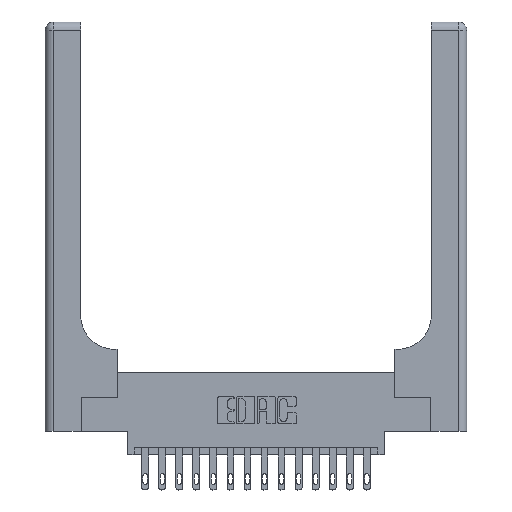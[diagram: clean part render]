
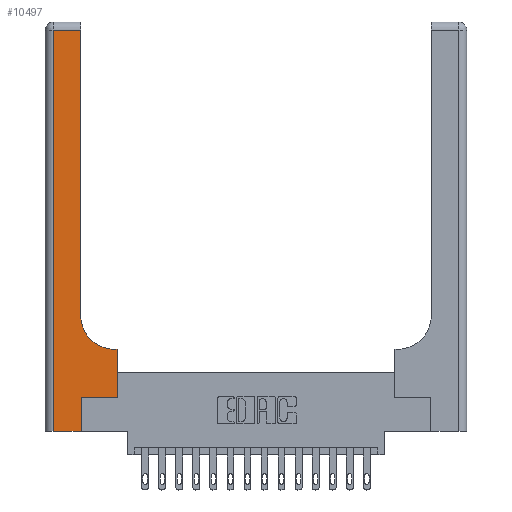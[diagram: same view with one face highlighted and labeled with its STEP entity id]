
A CAD part, top view. The second image highlights one B-rep face of the part: STEP entity #10497.
In plain terms, the highlighted planar face has unit normal (0, 0, 1).
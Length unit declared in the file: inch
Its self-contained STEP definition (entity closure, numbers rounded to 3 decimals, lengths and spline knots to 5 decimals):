
#294 = DIRECTION ( 'NONE',  ( -1., 0., 0. ) ) ;
#626 = LINE ( 'NONE', #2145, #14261 ) ;
#1012 = EDGE_CURVE ( 'NONE', #3552, #9337, #626, .T. ) ;
#1110 = VERTEX_POINT ( 'NONE', #9765 ) ;
#1452 = EDGE_CURVE ( 'NONE', #13508, #1110, #2634, .T. ) ;
#1680 = VECTOR ( 'NONE', #11181, 39.37008 ) ;
#2010 = EDGE_CURVE ( 'NONE', #9337, #5900, #4850, .T. ) ;
#2100 = VECTOR ( 'NONE', #17660, 39.37008 ) ;
#2145 = CARTESIAN_POINT ( 'NONE',  ( 0.06, 3., 0.37 ) ) ;
#2224 = AXIS2_PLACEMENT_3D ( 'NONE', #9870, #9687, #8454 ) ;
#2429 = CARTESIAN_POINT ( 'NONE',  ( 0., 3., 0.37 ) ) ;
#2634 = LINE ( 'NONE', #2726, #1680 ) ;
#2726 = CARTESIAN_POINT ( 'NONE',  ( 0.528, 0.25, 0.37 ) ) ;
#2947 = CARTESIAN_POINT ( 'NONE',  ( 0., 2.94, 0.37 ) ) ;
#3294 = VECTOR ( 'NONE', #8867, 39.37008 ) ;
#3315 = DIRECTION ( 'NONE',  ( -1., 0., 0. ) ) ;
#3552 = VERTEX_POINT ( 'NONE', #4098 ) ;
#3601 = CARTESIAN_POINT ( 'NONE',  ( 0.51, 0.6, 0.37 ) ) ;
#3669 = EDGE_CURVE ( 'NONE', #10164, #10861, #8691, .T. ) ;
#3693 = CARTESIAN_POINT ( 'NONE',  ( 0.26, 0.6, 0.37 ) ) ;
#4098 = CARTESIAN_POINT ( 'NONE',  ( 0.06, 2.94, 0.37 ) ) ;
#4128 = PLANE ( 'NONE',  #4860 ) ;
#4425 = CARTESIAN_POINT ( 'NONE',  ( 0.265, 0., 0.37 ) ) ;
#4574 = CARTESIAN_POINT ( 'NONE',  ( 0.265, 0.25, 0.37 ) ) ;
#4850 = LINE ( 'NONE', #15861, #9559 ) ;
#4860 = AXIS2_PLACEMENT_3D ( 'NONE', #2429, #15585, #13957 ) ;
#5301 = EDGE_CURVE ( 'NONE', #1110, #5337, #7560, .T. ) ;
#5337 = VERTEX_POINT ( 'NONE', #3601 ) ;
#5899 = EDGE_CURVE ( 'NONE', #11360, #13508, #14433, .T. ) ;
#5900 = VERTEX_POINT ( 'NONE', #10310 ) ;
#6257 = ORIENTED_EDGE ( 'NONE', *, *, #1012, .T. ) ;
#6306 = VECTOR ( 'NONE', #294, 39.37008 ) ;
#6399 = ORIENTED_EDGE ( 'NONE', *, *, #1452, .T. ) ;
#6915 = EDGE_LOOP ( 'NONE', ( #8743, #10645, #6257, #13335, #11617, #18460, #6399, #18344, #11744 ) ) ;
#7560 = LINE ( 'NONE', #3693, #11425 ) ;
#7671 = DIRECTION ( 'NONE',  ( 1., 0., 0. ) ) ;
#8454 = DIRECTION ( 'NONE',  ( 1., 0., 0. ) ) ;
#8691 = LINE ( 'NONE', #14410, #3294 ) ;
#8743 = ORIENTED_EDGE ( 'NONE', *, *, #3669, .T. ) ;
#8867 = DIRECTION ( 'NONE',  ( 0., 1., 0. ) ) ;
#9084 = CARTESIAN_POINT ( 'NONE',  ( 0.528, 0.25, 0.37 ) ) ;
#9337 = VERTEX_POINT ( 'NONE', #11596 ) ;
#9559 = VECTOR ( 'NONE', #10400, 39.37008 ) ;
#9687 = DIRECTION ( 'NONE',  ( 0., 0., -1. ) ) ;
#9765 = CARTESIAN_POINT ( 'NONE',  ( 0.528, 0.6, 0.37 ) ) ;
#9870 = CARTESIAN_POINT ( 'NONE',  ( 0.51, 0.85, 0.37 ) ) ;
#10066 = CARTESIAN_POINT ( 'NONE',  ( 0.265, 0.25, 0.37 ) ) ;
#10164 = VERTEX_POINT ( 'NONE', #10249 ) ;
#10249 = CARTESIAN_POINT ( 'NONE',  ( 0.26, 0.85, 0.37 ) ) ;
#10310 = CARTESIAN_POINT ( 'NONE',  ( 0.265, 0., 0.37 ) ) ;
#10342 = CIRCLE ( 'NONE', #2224, 0.25 ) ;
#10400 = DIRECTION ( 'NONE',  ( 1., 0., 0. ) ) ;
#10497 = ADVANCED_FACE ( 'NONE', ( #12645 ), #4128, .F. ) ;
#10645 = ORIENTED_EDGE ( 'NONE', *, *, #12958, .T. ) ;
#10861 = VERTEX_POINT ( 'NONE', #13758 ) ;
#11181 = DIRECTION ( 'NONE',  ( 0., 1., 0. ) ) ;
#11360 = VERTEX_POINT ( 'NONE', #10066 ) ;
#11425 = VECTOR ( 'NONE', #3315, 39.37008 ) ;
#11560 = EDGE_CURVE ( 'NONE', #5900, #11360, #13310, .T. ) ;
#11596 = CARTESIAN_POINT ( 'NONE',  ( 0.06, 0., 0.37 ) ) ;
#11617 = ORIENTED_EDGE ( 'NONE', *, *, #11560, .T. ) ;
#11744 = ORIENTED_EDGE ( 'NONE', *, *, #16178, .T. ) ;
#12645 = FACE_OUTER_BOUND ( 'NONE', #6915, .T. ) ;
#12958 = EDGE_CURVE ( 'NONE', #10861, #3552, #17139, .T. ) ;
#13310 = LINE ( 'NONE', #4425, #2100 ) ;
#13335 = ORIENTED_EDGE ( 'NONE', *, *, #2010, .T. ) ;
#13508 = VERTEX_POINT ( 'NONE', #9084 ) ;
#13679 = DIRECTION ( 'NONE',  ( 0., -1., 0. ) ) ;
#13758 = CARTESIAN_POINT ( 'NONE',  ( 0.26, 2.94, 0.37 ) ) ;
#13957 = DIRECTION ( 'NONE',  ( -1., 0., 0. ) ) ;
#14261 = VECTOR ( 'NONE', #13679, 39.37008 ) ;
#14410 = CARTESIAN_POINT ( 'NONE',  ( 0.26, 3., 0.37 ) ) ;
#14433 = LINE ( 'NONE', #4574, #16960 ) ;
#15585 = DIRECTION ( 'NONE',  ( 0., 0., -1. ) ) ;
#15861 = CARTESIAN_POINT ( 'NONE',  ( 0., 0., 0.37 ) ) ;
#16178 = EDGE_CURVE ( 'NONE', #5337, #10164, #10342, .T. ) ;
#16960 = VECTOR ( 'NONE', #7671, 39.37008 ) ;
#17139 = LINE ( 'NONE', #2947, #6306 ) ;
#17660 = DIRECTION ( 'NONE',  ( 0., 1., 0. ) ) ;
#18344 = ORIENTED_EDGE ( 'NONE', *, *, #5301, .T. ) ;
#18460 = ORIENTED_EDGE ( 'NONE', *, *, #5899, .T. ) ;
